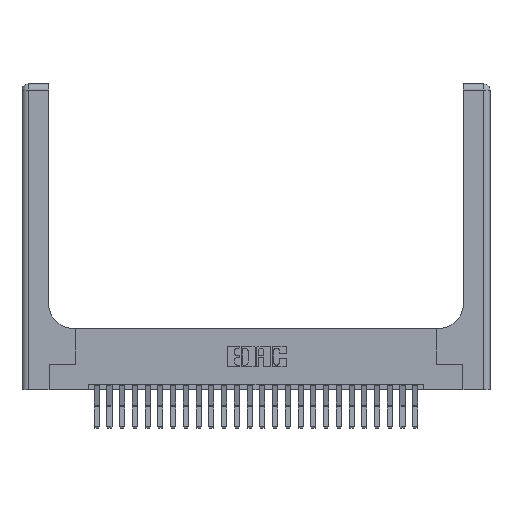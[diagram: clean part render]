
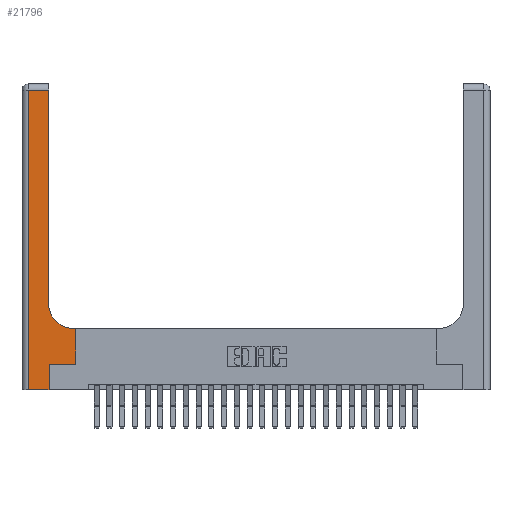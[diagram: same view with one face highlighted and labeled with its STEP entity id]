
A CAD part, top view. The second image highlights one B-rep face of the part: STEP entity #21796.
In plain terms, the highlighted planar face has unit normal (0, 0, 1).
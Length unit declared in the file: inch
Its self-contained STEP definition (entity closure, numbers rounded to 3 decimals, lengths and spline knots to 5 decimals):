
#34 = EDGE_CURVE ( 'NONE', #17596, #18363, #19069, .T. ) ;
#620 = DIRECTION ( 'NONE',  ( 0., 1., 0. ) ) ;
#720 = CARTESIAN_POINT ( 'NONE',  ( 0.26, 0.6, 0.37 ) ) ;
#930 = LINE ( 'NONE', #21367, #2403 ) ;
#1085 = AXIS2_PLACEMENT_3D ( 'NONE', #4684, #6344, #8231 ) ;
#1230 = CARTESIAN_POINT ( 'NONE',  ( 0.265, 0.25, 0.37 ) ) ;
#2403 = VECTOR ( 'NONE', #620, 39.37008 ) ;
#3113 = DIRECTION ( 'NONE',  ( 1., 0., 0. ) ) ;
#3188 = ORIENTED_EDGE ( 'NONE', *, *, #34, .T. ) ;
#3304 = ORIENTED_EDGE ( 'NONE', *, *, #18054, .T. ) ;
#3997 = VERTEX_POINT ( 'NONE', #15674 ) ;
#4115 = ORIENTED_EDGE ( 'NONE', *, *, #5945, .T. ) ;
#4684 = CARTESIAN_POINT ( 'NONE',  ( 0., 3., 0.37 ) ) ;
#4749 = ORIENTED_EDGE ( 'NONE', *, *, #11156, .T. ) ;
#5319 = CIRCLE ( 'NONE', #13979, 0.25 ) ;
#5349 = EDGE_CURVE ( 'NONE', #13907, #11648, #11704, .T. ) ;
#5608 = LINE ( 'NONE', #10951, #23640 ) ;
#5945 = EDGE_CURVE ( 'NONE', #12338, #6324, #18842, .T. ) ;
#6324 = VERTEX_POINT ( 'NONE', #13508 ) ;
#6344 = DIRECTION ( 'NONE',  ( 0., 0., -1. ) ) ;
#6518 = ORIENTED_EDGE ( 'NONE', *, *, #5349, .T. ) ;
#6785 = DIRECTION ( 'NONE',  ( 0., -1., 0. ) ) ;
#7582 = EDGE_CURVE ( 'NONE', #11648, #17596, #17225, .T. ) ;
#7687 = DIRECTION ( 'NONE',  ( 0., 1., 0. ) ) ;
#7782 = LINE ( 'NONE', #10502, #14536 ) ;
#8231 = DIRECTION ( 'NONE',  ( -1., 0., 0. ) ) ;
#9873 = CARTESIAN_POINT ( 'NONE',  ( 0.26, 0.85, 0.37 ) ) ;
#9959 = DIRECTION ( 'NONE',  ( 1., 0., 0. ) ) ;
#10205 = ORIENTED_EDGE ( 'NONE', *, *, #15221, .T. ) ;
#10226 = VECTOR ( 'NONE', #6785, 39.37008 ) ;
#10502 = CARTESIAN_POINT ( 'NONE',  ( 0., 0., 0.37 ) ) ;
#10718 = DIRECTION ( 'NONE',  ( 0., 1., 0. ) ) ;
#10951 = CARTESIAN_POINT ( 'NONE',  ( 0., 2.94, 0.37 ) ) ;
#11156 = EDGE_CURVE ( 'NONE', #21085, #3997, #930, .T. ) ;
#11648 = VERTEX_POINT ( 'NONE', #15959 ) ;
#11704 = LINE ( 'NONE', #1230, #12004 ) ;
#11786 = DIRECTION ( 'NONE',  ( -1., 0., 0. ) ) ;
#12004 = VECTOR ( 'NONE', #3113, 39.37008 ) ;
#12338 = VERTEX_POINT ( 'NONE', #23336 ) ;
#12605 = VECTOR ( 'NONE', #7687, 39.37008 ) ;
#12673 = CARTESIAN_POINT ( 'NONE',  ( 0.528, 0.25, 0.37 ) ) ;
#12689 = ORIENTED_EDGE ( 'NONE', *, *, #7582, .T. ) ;
#13058 = DIRECTION ( 'NONE',  ( -1., 0., 0. ) ) ;
#13508 = CARTESIAN_POINT ( 'NONE',  ( 0.06, 0., 0.37 ) ) ;
#13613 = CARTESIAN_POINT ( 'NONE',  ( 0.51, 0.6, 0.37 ) ) ;
#13904 = ORIENTED_EDGE ( 'NONE', *, *, #23880, .T. ) ;
#13907 = VERTEX_POINT ( 'NONE', #18157 ) ;
#13979 = AXIS2_PLACEMENT_3D ( 'NONE', #15559, #21267, #9959 ) ;
#14020 = VECTOR ( 'NONE', #11786, 39.37008 ) ;
#14536 = VECTOR ( 'NONE', #20082, 39.37008 ) ;
#15221 = EDGE_CURVE ( 'NONE', #6324, #18296, #7782, .T. ) ;
#15289 = CARTESIAN_POINT ( 'NONE',  ( 0.265, 0., 0.37 ) ) ;
#15559 = CARTESIAN_POINT ( 'NONE',  ( 0.51, 0.85, 0.37 ) ) ;
#15674 = CARTESIAN_POINT ( 'NONE',  ( 0.26, 2.94, 0.37 ) ) ;
#15959 = CARTESIAN_POINT ( 'NONE',  ( 0.528, 0.25, 0.37 ) ) ;
#17225 = LINE ( 'NONE', #12673, #24101 ) ;
#17596 = VERTEX_POINT ( 'NONE', #19454 ) ;
#18054 = EDGE_CURVE ( 'NONE', #3997, #12338, #5608, .T. ) ;
#18157 = CARTESIAN_POINT ( 'NONE',  ( 0.265, 0.25, 0.37 ) ) ;
#18296 = VERTEX_POINT ( 'NONE', #15289 ) ;
#18363 = VERTEX_POINT ( 'NONE', #13613 ) ;
#18842 = LINE ( 'NONE', #23685, #10226 ) ;
#19069 = LINE ( 'NONE', #720, #14020 ) ;
#19338 = EDGE_CURVE ( 'NONE', #18296, #13907, #22422, .T. ) ;
#19360 = ORIENTED_EDGE ( 'NONE', *, *, #19338, .T. ) ;
#19454 = CARTESIAN_POINT ( 'NONE',  ( 0.528, 0.6, 0.37 ) ) ;
#20082 = DIRECTION ( 'NONE',  ( 1., 0., 0. ) ) ;
#20695 = CARTESIAN_POINT ( 'NONE',  ( 0.265, 0., 0.37 ) ) ;
#21085 = VERTEX_POINT ( 'NONE', #9873 ) ;
#21267 = DIRECTION ( 'NONE',  ( 0., 0., -1. ) ) ;
#21367 = CARTESIAN_POINT ( 'NONE',  ( 0.26, 3., 0.37 ) ) ;
#21672 = PLANE ( 'NONE',  #1085 ) ;
#21796 = ADVANCED_FACE ( 'NONE', ( #22228 ), #21672, .F. ) ;
#22228 = FACE_OUTER_BOUND ( 'NONE', #23854, .T. ) ;
#22422 = LINE ( 'NONE', #20695, #12605 ) ;
#23336 = CARTESIAN_POINT ( 'NONE',  ( 0.06, 2.94, 0.37 ) ) ;
#23640 = VECTOR ( 'NONE', #13058, 39.37008 ) ;
#23685 = CARTESIAN_POINT ( 'NONE',  ( 0.06, 3., 0.37 ) ) ;
#23854 = EDGE_LOOP ( 'NONE', ( #4749, #3304, #4115, #10205, #19360, #6518, #12689, #3188, #13904 ) ) ;
#23880 = EDGE_CURVE ( 'NONE', #18363, #21085, #5319, .T. ) ;
#24101 = VECTOR ( 'NONE', #10718, 39.37008 ) ;
